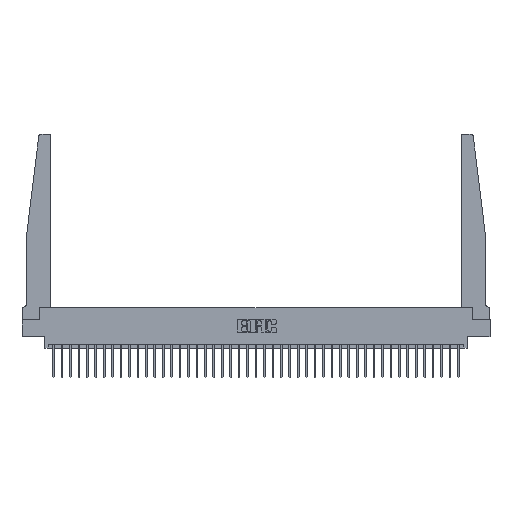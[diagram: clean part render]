
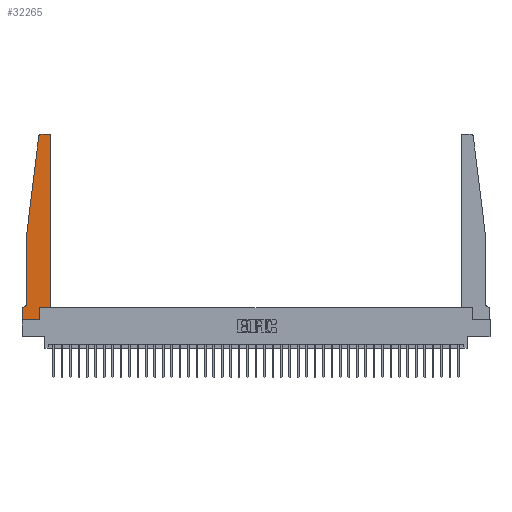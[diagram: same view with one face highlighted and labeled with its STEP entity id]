
A CAD part, top view. The second image highlights one B-rep face of the part: STEP entity #32265.
In plain terms, the highlighted planar face has unit normal (0, 0, 1).
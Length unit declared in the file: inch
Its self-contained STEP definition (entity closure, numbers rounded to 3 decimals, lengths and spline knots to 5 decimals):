
#646 = CARTESIAN_POINT ( 'NONE',  ( 0.2605, 0.18, 0.37 ) ) ;
#1440 = DIRECTION ( 'NONE',  ( -1., 0., 0. ) ) ;
#1532 = CARTESIAN_POINT ( 'NONE',  ( 0., 0., 0.37 ) ) ;
#1646 = CARTESIAN_POINT ( 'NONE',  ( 0.2605, 0., 0.37 ) ) ;
#2062 = CARTESIAN_POINT ( 'NONE',  ( 0.015, 0.1875, 0.37 ) ) ;
#2068 = EDGE_CURVE ( 'NONE', #22270, #2716, #21827, .T. ) ;
#2136 = AXIS2_PLACEMENT_3D ( 'NONE', #36051, #30679, #5617 ) ;
#2382 = EDGE_CURVE ( 'NONE', #33991, #25840, #3367, .T. ) ;
#2674 = VECTOR ( 'NONE', #30073, 39.37008 ) ;
#2695 = VECTOR ( 'NONE', #4675, 39.37008 ) ;
#2716 = VERTEX_POINT ( 'NONE', #16235 ) ;
#3163 = CARTESIAN_POINT ( 'NONE',  ( 0., 0.1875, 0.37 ) ) ;
#3356 = CARTESIAN_POINT ( 'NONE',  ( 0.425, 2.72, 0.37 ) ) ;
#3367 = LINE ( 'NONE', #26384, #20392 ) ;
#3757 = VERTEX_POINT ( 'NONE', #6493 ) ;
#3776 = LINE ( 'NONE', #646, #25395 ) ;
#4091 = ORIENTED_EDGE ( 'NONE', *, *, #8577, .T. ) ;
#4209 = CARTESIAN_POINT ( 'NONE',  ( 0.015, 0.2375, 0.37 ) ) ;
#4675 = DIRECTION ( 'NONE',  ( -1., 0., 0. ) ) ;
#4820 = VERTEX_POINT ( 'NONE', #1646 ) ;
#4858 = EDGE_CURVE ( 'NONE', #20612, #26750, #24326, .T. ) ;
#5268 = ORIENTED_EDGE ( 'NONE', *, *, #2068, .T. ) ;
#5617 = DIRECTION ( 'NONE',  ( 1., 0., 0. ) ) ;
#6166 = VERTEX_POINT ( 'NONE', #30056 ) ;
#6387 = CARTESIAN_POINT ( 'NONE',  ( 0., 0.1875, 0.37 ) ) ;
#6464 = CARTESIAN_POINT ( 'NONE',  ( 0.065, 1.25, 0.37 ) ) ;
#6493 = CARTESIAN_POINT ( 'NONE',  ( 0., 0., 0.37 ) ) ;
#6669 = EDGE_CURVE ( 'NONE', #4820, #11719, #3776, .T. ) ;
#7539 = EDGE_CURVE ( 'NONE', #24885, #20612, #17150, .T. ) ;
#7584 = AXIS2_PLACEMENT_3D ( 'NONE', #4209, #26692, #1440 ) ;
#7758 = CARTESIAN_POINT ( 'NONE',  ( 0.425, 0.18, 0.37 ) ) ;
#7799 = VECTOR ( 'NONE', #19033, 39.37008 ) ;
#8577 = EDGE_CURVE ( 'NONE', #13635, #22270, #18014, .T. ) ;
#9207 = DIRECTION ( 'NONE',  ( -0.122, -0.992, 0. ) ) ;
#9499 = EDGE_CURVE ( 'NONE', #6166, #13635, #33003, .T. ) ;
#10604 = EDGE_CURVE ( 'NONE', #3757, #4820, #33368, .T. ) ;
#10669 = AXIS2_PLACEMENT_3D ( 'NONE', #15115, #12540, #23613 ) ;
#10839 = EDGE_CURVE ( 'NONE', #2716, #24885, #31245, .T. ) ;
#11083 = CARTESIAN_POINT ( 'NONE',  ( 0., 0., 0.37 ) ) ;
#11550 = ORIENTED_EDGE ( 'NONE', *, *, #10604, .T. ) ;
#11701 = DIRECTION ( 'NONE',  ( 0., 1., 0. ) ) ;
#11719 = VERTEX_POINT ( 'NONE', #11904 ) ;
#11725 = FACE_OUTER_BOUND ( 'NONE', #20752, .T. ) ;
#11904 = CARTESIAN_POINT ( 'NONE',  ( 0.2605, 0.18, 0.37 ) ) ;
#12327 = AXIS2_PLACEMENT_3D ( 'NONE', #6387, #25925, #31048 ) ;
#12353 = CARTESIAN_POINT ( 'NONE',  ( 0.24675, 2.72367, 0.37 ) ) ;
#12437 = VECTOR ( 'NONE', #16784, 39.37008 ) ;
#12520 = CARTESIAN_POINT ( 'NONE',  ( 0.395, 2.75, 0.37 ) ) ;
#12540 = DIRECTION ( 'NONE',  ( 0., 0., 1. ) ) ;
#13147 = CARTESIAN_POINT ( 'NONE',  ( 0.25, 2.75, 0.37 ) ) ;
#13306 = EDGE_CURVE ( 'NONE', #25840, #3757, #34520, .T. ) ;
#13635 = VERTEX_POINT ( 'NONE', #3356 ) ;
#13676 = CARTESIAN_POINT ( 'NONE',  ( 0.425, 0.18, 0.37 ) ) ;
#13734 = ORIENTED_EDGE ( 'NONE', *, *, #7539, .T. ) ;
#14981 = CARTESIAN_POINT ( 'NONE',  ( 0.065, 0.2375, 0.37 ) ) ;
#15115 = CARTESIAN_POINT ( 'NONE',  ( 0.27653, 2.72, 0.37 ) ) ;
#15388 = VECTOR ( 'NONE', #21557, 39.37008 ) ;
#15541 = DIRECTION ( 'NONE',  ( 0., -1., 0. ) ) ;
#15715 = LINE ( 'NONE', #13676, #2674 ) ;
#15968 = VECTOR ( 'NONE', #9207, 39.37008 ) ;
#16235 = CARTESIAN_POINT ( 'NONE',  ( 0.27653, 2.75, 0.37 ) ) ;
#16576 = CARTESIAN_POINT ( 'NONE',  ( 0.065, 1.25, 0.37 ) ) ;
#16589 = ORIENTED_EDGE ( 'NONE', *, *, #10839, .T. ) ;
#16784 = DIRECTION ( 'NONE',  ( 1., 0., 0. ) ) ;
#17063 = ORIENTED_EDGE ( 'NONE', *, *, #4858, .T. ) ;
#17150 = LINE ( 'NONE', #6464, #15968 ) ;
#18014 = CIRCLE ( 'NONE', #2136, 0.03 ) ;
#19033 = DIRECTION ( 'NONE',  ( 0., 1., 0. ) ) ;
#19864 = ORIENTED_EDGE ( 'NONE', *, *, #2382, .T. ) ;
#20392 = VECTOR ( 'NONE', #20503, 39.37008 ) ;
#20503 = DIRECTION ( 'NONE',  ( -1., 0., 0. ) ) ;
#20612 = VERTEX_POINT ( 'NONE', #16576 ) ;
#20752 = EDGE_LOOP ( 'NONE', ( #5268, #16589, #13734, #17063, #27311, #19864, #21647, #11550, #32995, #29626, #31809, #4091 ) ) ;
#21557 = DIRECTION ( 'NONE',  ( 0., -1., 0. ) ) ;
#21647 = ORIENTED_EDGE ( 'NONE', *, *, #13306, .T. ) ;
#21827 = LINE ( 'NONE', #13147, #2695 ) ;
#22270 = VERTEX_POINT ( 'NONE', #12520 ) ;
#23613 = DIRECTION ( 'NONE',  ( 1., 0., 0. ) ) ;
#24326 = LINE ( 'NONE', #35547, #15388 ) ;
#24885 = VERTEX_POINT ( 'NONE', #12353 ) ;
#25395 = VECTOR ( 'NONE', #11701, 39.37008 ) ;
#25679 = EDGE_CURVE ( 'NONE', #11719, #6166, #15715, .T. ) ;
#25840 = VERTEX_POINT ( 'NONE', #3163 ) ;
#25925 = DIRECTION ( 'NONE',  ( 0., 0., 1. ) ) ;
#26384 = CARTESIAN_POINT ( 'NONE',  ( 0.065, 0.1875, 0.37 ) ) ;
#26692 = DIRECTION ( 'NONE',  ( 0., 0., -1. ) ) ;
#26750 = VERTEX_POINT ( 'NONE', #14981 ) ;
#27311 = ORIENTED_EDGE ( 'NONE', *, *, #31969, .T. ) ;
#29626 = ORIENTED_EDGE ( 'NONE', *, *, #25679, .T. ) ;
#30056 = CARTESIAN_POINT ( 'NONE',  ( 0.425, 0.18, 0.37 ) ) ;
#30073 = DIRECTION ( 'NONE',  ( 1., 0., 0. ) ) ;
#30679 = DIRECTION ( 'NONE',  ( 0., 0., 1. ) ) ;
#31048 = DIRECTION ( 'NONE',  ( 1., 0., 0. ) ) ;
#31245 = CIRCLE ( 'NONE', #10669, 0.03 ) ;
#31809 = ORIENTED_EDGE ( 'NONE', *, *, #9499, .T. ) ;
#31874 = VECTOR ( 'NONE', #15541, 39.37008 ) ;
#31969 = EDGE_CURVE ( 'NONE', #26750, #33991, #33464, .T. ) ;
#32265 = ADVANCED_FACE ( 'NONE', ( #11725 ), #34375, .T. ) ;
#32995 = ORIENTED_EDGE ( 'NONE', *, *, #6669, .T. ) ;
#33003 = LINE ( 'NONE', #7758, #7799 ) ;
#33368 = LINE ( 'NONE', #11083, #12437 ) ;
#33464 = CIRCLE ( 'NONE', #7584, 0.05 ) ;
#33991 = VERTEX_POINT ( 'NONE', #2062 ) ;
#34375 = PLANE ( 'NONE',  #12327 ) ;
#34520 = LINE ( 'NONE', #1532, #31874 ) ;
#35547 = CARTESIAN_POINT ( 'NONE',  ( 0.065, 1.25, 0.37 ) ) ;
#36051 = CARTESIAN_POINT ( 'NONE',  ( 0.395, 2.72, 0.37 ) ) ;
